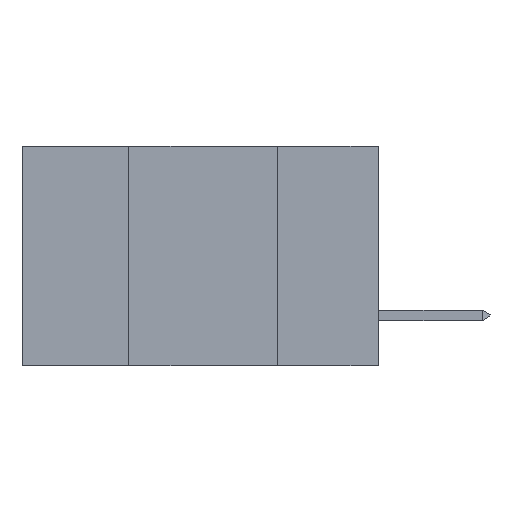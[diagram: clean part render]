
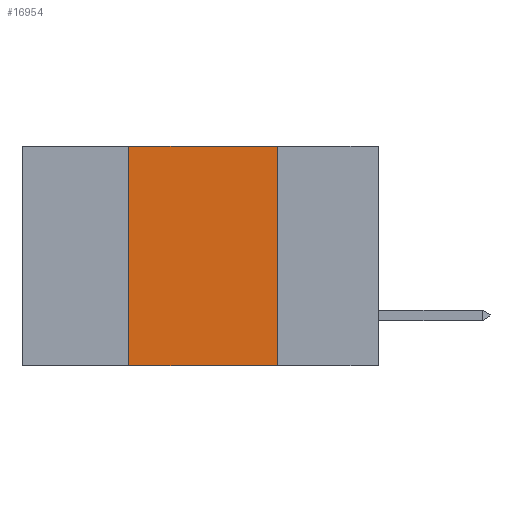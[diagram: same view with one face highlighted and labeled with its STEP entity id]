
A CAD part, left-side view. The second image highlights one B-rep face of the part: STEP entity #16954.
In plain terms, the highlighted planar face has unit normal (-1, 0, 0).
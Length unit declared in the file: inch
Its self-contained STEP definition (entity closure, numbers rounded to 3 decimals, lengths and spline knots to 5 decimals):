
#841 = VECTOR ( 'NONE', #24225, 39.37008 ) ;
#1055 = EDGE_CURVE ( 'NONE', #24504, #2156, #2155, .T. ) ;
#1481 = CARTESIAN_POINT ( 'NONE',  ( 0., 0.17, -0.37 ) ) ;
#1578 = DIRECTION ( 'NONE',  ( 0., 0., -1. ) ) ;
#2155 = LINE ( 'NONE', #4719, #5702 ) ;
#2156 = VERTEX_POINT ( 'NONE', #5610 ) ;
#3399 = CARTESIAN_POINT ( 'NONE',  ( 0., 0.6, 0. ) ) ;
#3436 = AXIS2_PLACEMENT_3D ( 'NONE', #11246, #19898, #21806 ) ;
#3799 = LINE ( 'NONE', #19935, #841 ) ;
#4719 = CARTESIAN_POINT ( 'NONE',  ( 0., 0.42, 0. ) ) ;
#4951 = LINE ( 'NONE', #3399, #20374 ) ;
#5610 = CARTESIAN_POINT ( 'NONE',  ( 0., 0.42, 0. ) ) ;
#5702 = VECTOR ( 'NONE', #13402, 39.37008 ) ;
#6478 = EDGE_CURVE ( 'NONE', #24504, #23554, #3799, .T. ) ;
#6797 = ORIENTED_EDGE ( 'NONE', *, *, #19825, .F. ) ;
#8534 = VERTEX_POINT ( 'NONE', #9289 ) ;
#8607 = EDGE_LOOP ( 'NONE', ( #6797, #25937, #26429, #21958 ) ) ;
#9289 = CARTESIAN_POINT ( 'NONE',  ( 0., 0.17, 0. ) ) ;
#9716 = DIRECTION ( 'NONE',  ( 0., -1., 0. ) ) ;
#10165 = CARTESIAN_POINT ( 'NONE',  ( 0., 0.17, 0. ) ) ;
#11246 = CARTESIAN_POINT ( 'NONE',  ( 0., 0.6, 0. ) ) ;
#11407 = EDGE_CURVE ( 'NONE', #2156, #8534, #4951, .T. ) ;
#13402 = DIRECTION ( 'NONE',  ( 0., 0., 1. ) ) ;
#16954 = ADVANCED_FACE ( 'NONE', ( #23901 ), #19474, .F. ) ;
#17544 = CARTESIAN_POINT ( 'NONE',  ( 0., 0.42, -0.37 ) ) ;
#19474 = PLANE ( 'NONE',  #3436 ) ;
#19825 = EDGE_CURVE ( 'NONE', #8534, #23554, #21285, .T. ) ;
#19898 = DIRECTION ( 'NONE',  ( 1., 0., 0. ) ) ;
#19935 = CARTESIAN_POINT ( 'NONE',  ( 0., 0.6, -0.37 ) ) ;
#20374 = VECTOR ( 'NONE', #9716, 39.37008 ) ;
#21285 = LINE ( 'NONE', #10165, #22211 ) ;
#21806 = DIRECTION ( 'NONE',  ( 0., 0., -1. ) ) ;
#21958 = ORIENTED_EDGE ( 'NONE', *, *, #6478, .T. ) ;
#22211 = VECTOR ( 'NONE', #1578, 39.37008 ) ;
#23554 = VERTEX_POINT ( 'NONE', #1481 ) ;
#23901 = FACE_OUTER_BOUND ( 'NONE', #8607, .T. ) ;
#24225 = DIRECTION ( 'NONE',  ( 0., -1., 0. ) ) ;
#24504 = VERTEX_POINT ( 'NONE', #17544 ) ;
#25937 = ORIENTED_EDGE ( 'NONE', *, *, #11407, .F. ) ;
#26429 = ORIENTED_EDGE ( 'NONE', *, *, #1055, .F. ) ;
